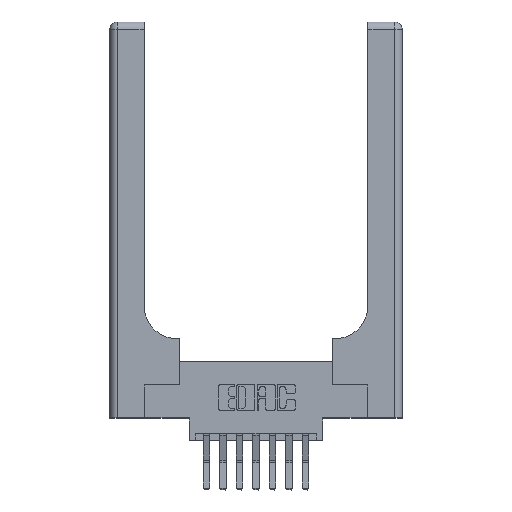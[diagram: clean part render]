
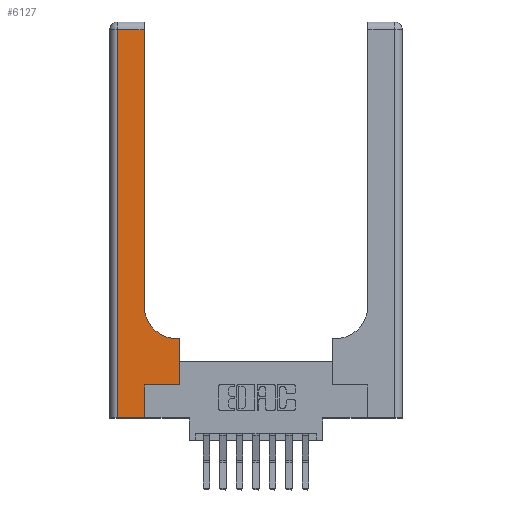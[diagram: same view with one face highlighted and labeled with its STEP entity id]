
A CAD part, top view. The second image highlights one B-rep face of the part: STEP entity #6127.
In plain terms, the highlighted planar face has unit normal (0, 0, 1).
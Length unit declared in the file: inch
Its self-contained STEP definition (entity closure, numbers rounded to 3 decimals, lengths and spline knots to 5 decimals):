
#74 = ORIENTED_EDGE ( 'NONE', *, *, #8907, .T. ) ;
#106 = AXIS2_PLACEMENT_3D ( 'NONE', #13871, #3391, #4314 ) ;
#288 = VECTOR ( 'NONE', #9740, 39.37008 ) ;
#428 = CIRCLE ( 'NONE', #10941, 0.25 ) ;
#693 = CARTESIAN_POINT ( 'NONE',  ( 0.26, 3., 0.37 ) ) ;
#814 = LINE ( 'NONE', #13813, #14280 ) ;
#943 = PLANE ( 'NONE',  #106 ) ;
#1041 = LINE ( 'NONE', #4553, #5802 ) ;
#1212 = CARTESIAN_POINT ( 'NONE',  ( 0.51, 0.85, 0.37 ) ) ;
#1251 = ORIENTED_EDGE ( 'NONE', *, *, #5737, .T. ) ;
#1588 = VECTOR ( 'NONE', #5511, 39.37008 ) ;
#1686 = VECTOR ( 'NONE', #3731, 39.37008 ) ;
#1843 = VECTOR ( 'NONE', #11550, 39.37008 ) ;
#2183 = DIRECTION ( 'NONE',  ( 1., 0., 0. ) ) ;
#2738 = VERTEX_POINT ( 'NONE', #4284 ) ;
#2790 = ORIENTED_EDGE ( 'NONE', *, *, #14081, .T. ) ;
#3197 = DIRECTION ( 'NONE',  ( 0., -1., 0. ) ) ;
#3287 = CARTESIAN_POINT ( 'NONE',  ( 0.528, 0.25, 0.37 ) ) ;
#3391 = DIRECTION ( 'NONE',  ( 0., 0., -1. ) ) ;
#3731 = DIRECTION ( 'NONE',  ( 0., 1., 0. ) ) ;
#4160 = EDGE_CURVE ( 'NONE', #14868, #12290, #1041, .T. ) ;
#4284 = CARTESIAN_POINT ( 'NONE',  ( 0.26, 0.85, 0.37 ) ) ;
#4314 = DIRECTION ( 'NONE',  ( -1., 0., 0. ) ) ;
#4418 = DIRECTION ( 'NONE',  ( 0., 0., -1. ) ) ;
#4553 = CARTESIAN_POINT ( 'NONE',  ( 0.06, 3., 0.37 ) ) ;
#4665 = CARTESIAN_POINT ( 'NONE',  ( 0.06, 0., 0.37 ) ) ;
#4717 = DIRECTION ( 'NONE',  ( 1., 0., 0. ) ) ;
#4793 = LINE ( 'NONE', #13835, #1843 ) ;
#4916 = ORIENTED_EDGE ( 'NONE', *, *, #6488, .T. ) ;
#5013 = CARTESIAN_POINT ( 'NONE',  ( 0.265, 0., 0.37 ) ) ;
#5288 = CARTESIAN_POINT ( 'NONE',  ( 0.265, 0., 0.37 ) ) ;
#5488 = CARTESIAN_POINT ( 'NONE',  ( 0.528, 0.25, 0.37 ) ) ;
#5511 = DIRECTION ( 'NONE',  ( -1., 0., 0. ) ) ;
#5737 = EDGE_CURVE ( 'NONE', #12290, #9952, #814, .T. ) ;
#5802 = VECTOR ( 'NONE', #3197, 39.37008 ) ;
#6032 = ORIENTED_EDGE ( 'NONE', *, *, #13262, .T. ) ;
#6127 = ADVANCED_FACE ( 'NONE', ( #14795 ), #943, .F. ) ;
#6317 = CARTESIAN_POINT ( 'NONE',  ( 0.06, 2.94, 0.37 ) ) ;
#6488 = EDGE_CURVE ( 'NONE', #6585, #6632, #10125, .T. ) ;
#6585 = VERTEX_POINT ( 'NONE', #7041 ) ;
#6632 = VERTEX_POINT ( 'NONE', #15074 ) ;
#6949 = EDGE_CURVE ( 'NONE', #7414, #14529, #4793, .T. ) ;
#7041 = CARTESIAN_POINT ( 'NONE',  ( 0.528, 0.6, 0.37 ) ) ;
#7110 = VECTOR ( 'NONE', #13768, 39.37008 ) ;
#7414 = VERTEX_POINT ( 'NONE', #13497 ) ;
#8081 = DIRECTION ( 'NONE',  ( -1., 0., 0. ) ) ;
#8142 = EDGE_LOOP ( 'NONE', ( #12564, #9929, #8353, #1251, #6032, #12029, #2790, #4916, #74 ) ) ;
#8175 = LINE ( 'NONE', #3287, #7110 ) ;
#8353 = ORIENTED_EDGE ( 'NONE', *, *, #4160, .T. ) ;
#8480 = EDGE_CURVE ( 'NONE', #11238, #14868, #13905, .T. ) ;
#8727 = LINE ( 'NONE', #693, #288 ) ;
#8907 = EDGE_CURVE ( 'NONE', #6632, #2738, #428, .T. ) ;
#9740 = DIRECTION ( 'NONE',  ( 0., 1., 0. ) ) ;
#9929 = ORIENTED_EDGE ( 'NONE', *, *, #8480, .T. ) ;
#9952 = VERTEX_POINT ( 'NONE', #5288 ) ;
#10125 = LINE ( 'NONE', #12339, #1588 ) ;
#10941 = AXIS2_PLACEMENT_3D ( 'NONE', #1212, #4418, #4717 ) ;
#11238 = VERTEX_POINT ( 'NONE', #13347 ) ;
#11550 = DIRECTION ( 'NONE',  ( 1., 0., 0. ) ) ;
#11644 = EDGE_CURVE ( 'NONE', #2738, #11238, #8727, .T. ) ;
#11691 = CARTESIAN_POINT ( 'NONE',  ( 0., 2.94, 0.37 ) ) ;
#12029 = ORIENTED_EDGE ( 'NONE', *, *, #6949, .T. ) ;
#12290 = VERTEX_POINT ( 'NONE', #4665 ) ;
#12339 = CARTESIAN_POINT ( 'NONE',  ( 0.26, 0.6, 0.37 ) ) ;
#12564 = ORIENTED_EDGE ( 'NONE', *, *, #11644, .T. ) ;
#12988 = LINE ( 'NONE', #5013, #1686 ) ;
#13262 = EDGE_CURVE ( 'NONE', #9952, #7414, #12988, .T. ) ;
#13347 = CARTESIAN_POINT ( 'NONE',  ( 0.26, 2.94, 0.37 ) ) ;
#13497 = CARTESIAN_POINT ( 'NONE',  ( 0.265, 0.25, 0.37 ) ) ;
#13768 = DIRECTION ( 'NONE',  ( 0., 1., 0. ) ) ;
#13813 = CARTESIAN_POINT ( 'NONE',  ( 0., 0., 0.37 ) ) ;
#13835 = CARTESIAN_POINT ( 'NONE',  ( 0.265, 0.25, 0.37 ) ) ;
#13871 = CARTESIAN_POINT ( 'NONE',  ( 0., 3., 0.37 ) ) ;
#13905 = LINE ( 'NONE', #11691, #14830 ) ;
#14081 = EDGE_CURVE ( 'NONE', #14529, #6585, #8175, .T. ) ;
#14280 = VECTOR ( 'NONE', #2183, 39.37008 ) ;
#14529 = VERTEX_POINT ( 'NONE', #5488 ) ;
#14795 = FACE_OUTER_BOUND ( 'NONE', #8142, .T. ) ;
#14830 = VECTOR ( 'NONE', #8081, 39.37008 ) ;
#14868 = VERTEX_POINT ( 'NONE', #6317 ) ;
#15074 = CARTESIAN_POINT ( 'NONE',  ( 0.51, 0.6, 0.37 ) ) ;
